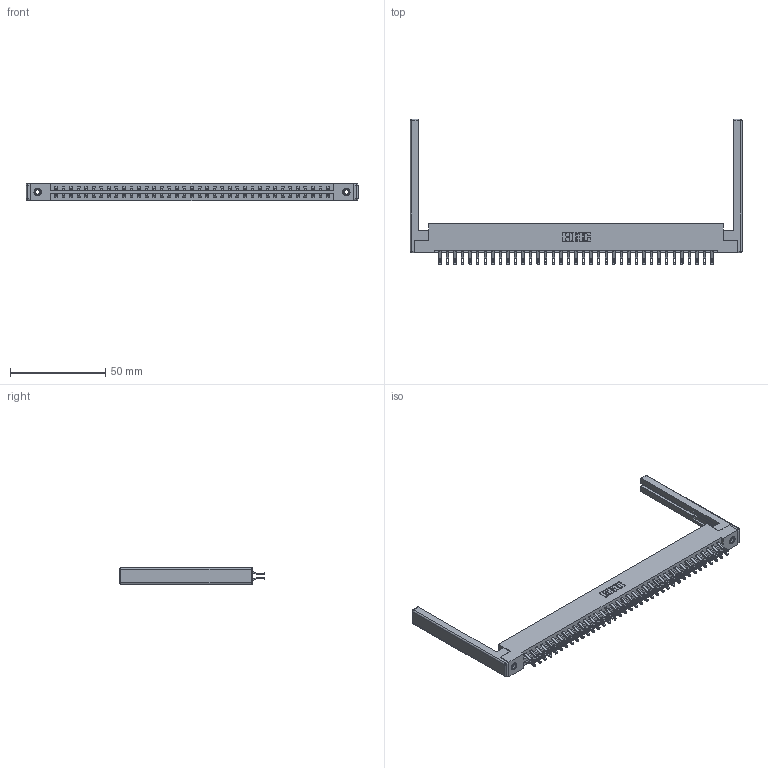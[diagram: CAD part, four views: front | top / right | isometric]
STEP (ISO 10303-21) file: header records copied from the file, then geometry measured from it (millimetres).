
FILE_DESCRIPTION (( 'STEP AP203' ), '1' );
FILE_NAME ('337-074-555-268.STEP', '2019-10-10T04:09:08', ( '' ), ( '' ), 'SwSTEP 2.0', 'SolidWorks 2016', '' );
FILE_SCHEMA (( 'CONFIG_CONTROL_DESIGN' ));
Length unit declared in the file: inch
Products named in the file (5): 345-250-001_345-250-001-102; 345-292-001_555 Tail; 337-074-555-268; 307-220-068; 337 Part_Flush Mounting Lugs - 0.156 Dia-TI
Assembly tree (79 placements, depth 2):
  337-074-555-268
    337 Part_Flush Mounting Lugs - 0.156 Dia-TI
    345-292-001_555 Tail  x74
    345-250-001_345-250-001-102  x2
    307-220-068  x2
Bounding box: 174.04 x 76.21 x 9.4 mm (x, y, z)
Volume: 22874.7 mm3; surface area: 25697.5 mm2
Topology: 79 solids, 79 shells, 4708 faces, 14687 edges, 9770 vertices
Faces by surface type: plane 2822, cylinder 1862, cone 12, sphere 8, torus 4
Entity records: 32420 total; most frequent: CARTESIAN_POINT 5465, ORIENTED_EDGE 5360, DIRECTION 4698, EDGE_CURVE 2680, LINE 2482, VECTOR 2482, VERTEX_POINT 1778, AXIS2_PLACEMENT_3D 1108
